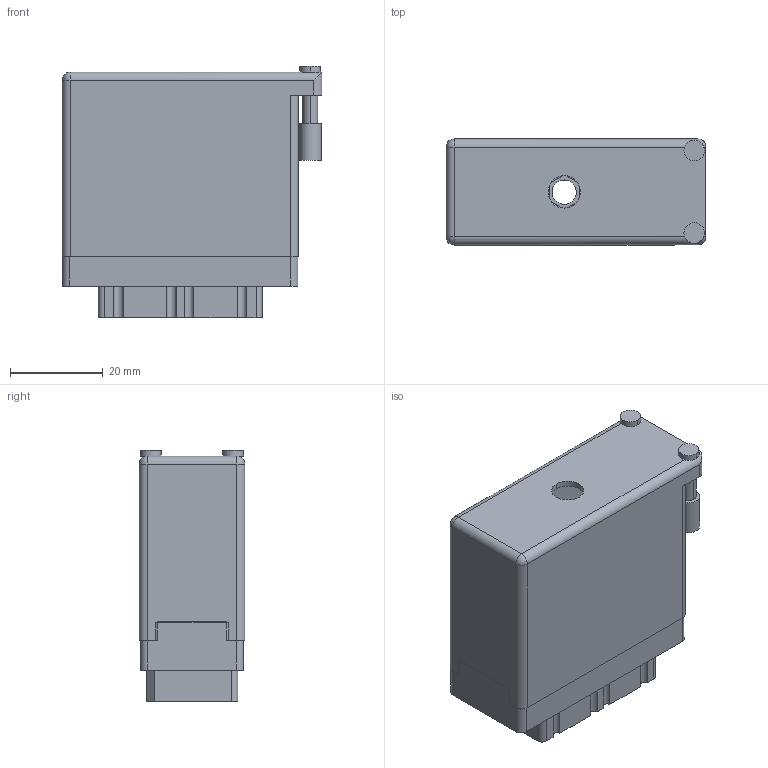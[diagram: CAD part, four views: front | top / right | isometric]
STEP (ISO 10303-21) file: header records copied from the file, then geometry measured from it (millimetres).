
FILE_DESCRIPTION (( 'STEP AP203' ), '1' );
FILE_NAME ('519-036-000-450.STEP', '2020-09-09T20:01:42', ( '' ), ( '' ), 'SwSTEP 2.0', 'SolidWorks 2020', '' );
FILE_SCHEMA (( 'CONFIG_CONTROL_DESIGN' ));
Length unit declared in the file: inch
Products named in the file (3): 516-230-001_Metal - 038 Side Entry; 519 Receptacle Insulator_036; 519-036-000-450
Assembly tree (2 placements, depth 2):
  519-036-000-450
    519 Receptacle Insulator_036
    516-230-001_Metal - 038 Side Entry
Bounding box: 56.08 x 22.83 x 54.28 mm (x, y, z)
Volume: 19883.6 mm3; surface area: 27577.1 mm2
Topology: 2 solids, 2 shells, 909 faces, 2650 edges, 1760 vertices
Faces by surface type: plane 644, cylinder 261, cone 2, sphere 2
Entity records: 30561 total; most frequent: CARTESIAN_POINT 5363, ORIENTED_EDGE 5296, DIRECTION 5134, EDGE_CURVE 2648, VECTOR 1980, LINE 1980, VERTEX_POINT 1760, AXIS2_PLACEMENT_3D 1577
